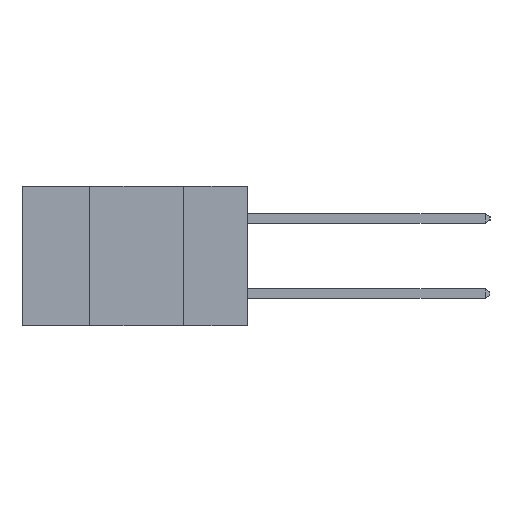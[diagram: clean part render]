
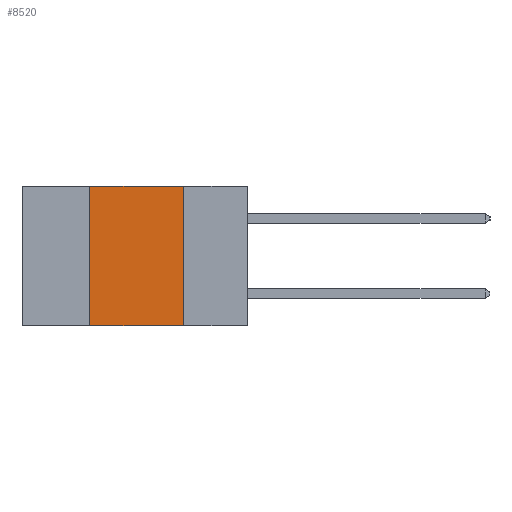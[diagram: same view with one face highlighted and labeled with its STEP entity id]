
A CAD part, left-side view. The second image highlights one B-rep face of the part: STEP entity #8520.
In plain terms, the highlighted planar face has unit normal (-1, 0, 0).
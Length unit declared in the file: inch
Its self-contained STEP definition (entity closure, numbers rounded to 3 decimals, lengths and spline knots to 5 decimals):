
#1455 = DIRECTION ( 'NONE',  ( 0., -1., 0. ) ) ;
#4132 = CARTESIAN_POINT ( 'NONE',  ( 0., 0.17, -0.37 ) ) ;
#4841 = CARTESIAN_POINT ( 'NONE',  ( 0., 0.42, -0.37 ) ) ;
#6031 = AXIS2_PLACEMENT_3D ( 'NONE', #10291, #24603, #12363 ) ;
#6261 = DIRECTION ( 'NONE',  ( 0., 0., -1. ) ) ;
#6730 = LINE ( 'NONE', #20084, #12217 ) ;
#6970 = DIRECTION ( 'NONE',  ( 0., 0., 1. ) ) ;
#7842 = EDGE_CURVE ( 'NONE', #17268, #25490, #13313, .T. ) ;
#8520 = ADVANCED_FACE ( 'NONE', ( #12947 ), #22453, .F. ) ;
#8809 = ORIENTED_EDGE ( 'NONE', *, *, #7842, .F. ) ;
#10291 = CARTESIAN_POINT ( 'NONE',  ( 0., 0.6, 0. ) ) ;
#10372 = VERTEX_POINT ( 'NONE', #17408 ) ;
#10998 = VECTOR ( 'NONE', #14385, 39.37008 ) ;
#12217 = VECTOR ( 'NONE', #1455, 39.37008 ) ;
#12325 = CARTESIAN_POINT ( 'NONE',  ( 0., 0.6, -0.37 ) ) ;
#12363 = DIRECTION ( 'NONE',  ( 0., 0., -1. ) ) ;
#12915 = EDGE_CURVE ( 'NONE', #16784, #10372, #24821, .T. ) ;
#12947 = FACE_OUTER_BOUND ( 'NONE', #25440, .T. ) ;
#13020 = ORIENTED_EDGE ( 'NONE', *, *, #12915, .F. ) ;
#13313 = LINE ( 'NONE', #4132, #23513 ) ;
#13956 = VECTOR ( 'NONE', #6970, 39.37008 ) ;
#14385 = DIRECTION ( 'NONE',  ( 0., -1., 0. ) ) ;
#16445 = LINE ( 'NONE', #12325, #10998 ) ;
#16784 = VERTEX_POINT ( 'NONE', #21144 ) ;
#17268 = VERTEX_POINT ( 'NONE', #22539 ) ;
#17294 = CARTESIAN_POINT ( 'NONE',  ( 0., 0.17, -0.37 ) ) ;
#17408 = CARTESIAN_POINT ( 'NONE',  ( 0., 0.42, 0. ) ) ;
#20084 = CARTESIAN_POINT ( 'NONE',  ( 0., 0.6, 0. ) ) ;
#21144 = CARTESIAN_POINT ( 'NONE',  ( 0., 0.42, -0.37 ) ) ;
#21950 = ORIENTED_EDGE ( 'NONE', *, *, #23846, .T. ) ;
#22453 = PLANE ( 'NONE',  #6031 ) ;
#22539 = CARTESIAN_POINT ( 'NONE',  ( 0., 0.17, 0. ) ) ;
#23513 = VECTOR ( 'NONE', #6261, 39.37008 ) ;
#23846 = EDGE_CURVE ( 'NONE', #16784, #25490, #16445, .T. ) ;
#24497 = ORIENTED_EDGE ( 'NONE', *, *, #25023, .F. ) ;
#24603 = DIRECTION ( 'NONE',  ( 1., 0., 0. ) ) ;
#24821 = LINE ( 'NONE', #4841, #13956 ) ;
#25023 = EDGE_CURVE ( 'NONE', #10372, #17268, #6730, .T. ) ;
#25440 = EDGE_LOOP ( 'NONE', ( #8809, #24497, #13020, #21950 ) ) ;
#25490 = VERTEX_POINT ( 'NONE', #17294 ) ;
